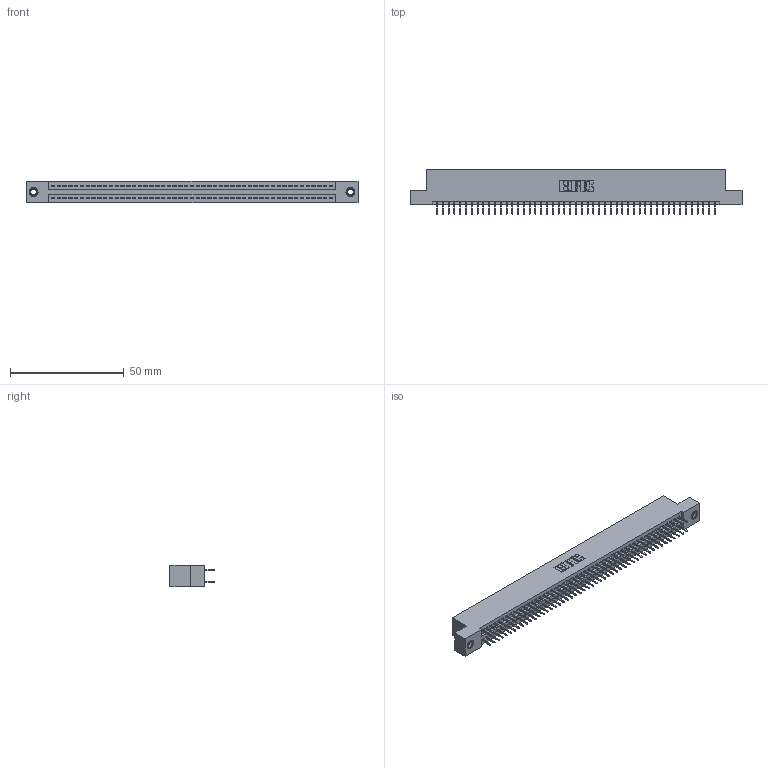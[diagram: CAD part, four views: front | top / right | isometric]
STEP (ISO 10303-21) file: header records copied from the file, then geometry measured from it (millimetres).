
FILE_DESCRIPTION (( 'STEP AP203' ), '1' );
FILE_NAME ('345-098-524-207.STEP', '2018-10-05T09:00:24', ( '' ), ( '' ), 'SwSTEP 2.0', 'SolidWorks 2016', '' );
FILE_SCHEMA (( 'CONFIG_CONTROL_DESIGN' ));
Length unit declared in the file: inch
Products named in the file (4): 345 Part_Flush Mounting Lugs - 0.156 Dia-TI; 345-250-001_345-250-005-103; 345-098-524-207; 345-292-001_345-293-124
Assembly tree (101 placements, depth 2):
  345-098-524-207
    345 Part_Flush Mounting Lugs - 0.156 Dia-TI
    345-292-001_345-293-124  x98
    345-250-001_345-250-005-103  x2
Bounding box: 145.67 x 19.35 x 9.4 mm (x, y, z)
Volume: 14053.6 mm3; surface area: 20545.5 mm2
Topology: 101 solids, 101 shells, 5478 faces, 15471 edges, 9914 vertices
Faces by surface type: plane 3934, cylinder 1528, cone 12, torus 4
Entity records: 38764 total; most frequent: CARTESIAN_POINT 6471, ORIENTED_EDGE 6398, DIRECTION 5725, EDGE_CURVE 3199, VECTOR 2855, LINE 2855, VERTEX_POINT 2124, AXIS2_PLACEMENT_3D 1435
